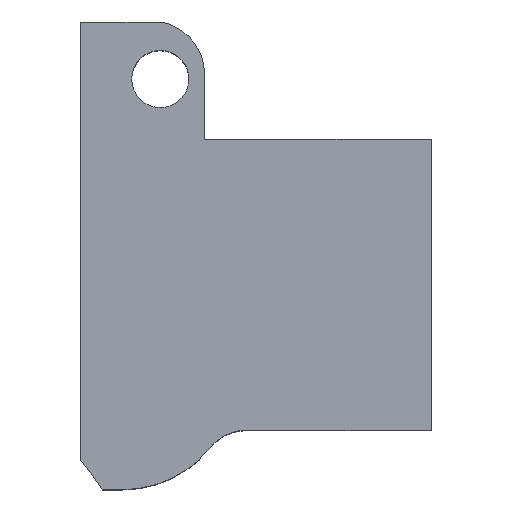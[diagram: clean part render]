
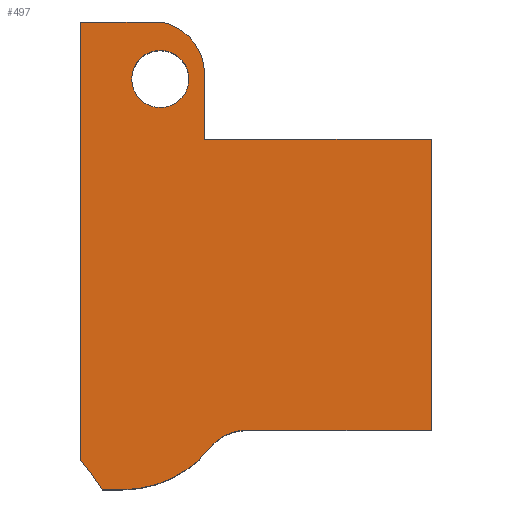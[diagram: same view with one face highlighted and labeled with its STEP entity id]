
A CAD part, top view. The second image highlights one B-rep face of the part: STEP entity #497.
In plain terms, the highlighted planar face has unit normal (0, 0, 1).
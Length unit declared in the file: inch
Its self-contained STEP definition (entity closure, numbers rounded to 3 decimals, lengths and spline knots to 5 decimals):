
#15 = FACE_OUTER_BOUND ( 'NONE', #800, .T. ) ;
#30 = CARTESIAN_POINT ( 'NONE',  ( 3.70038, -0.51472, 0.4665 ) ) ;
#53 = VERTEX_POINT ( 'NONE', #881 ) ;
#54 = CARTESIAN_POINT ( 'NONE',  ( 2.19337, -1.9664, 0.4665 ) ) ;
#58 = DIRECTION ( 'NONE',  ( 0., 0., -1. ) ) ;
#61 = DIRECTION ( 'NONE',  ( 0., -1., 0. ) ) ;
#66 = ORIENTED_EDGE ( 'NONE', *, *, #389, .T. ) ;
#77 = VECTOR ( 'NONE', #61, 39.37008 ) ;
#79 = AXIS2_PLACEMENT_3D ( 'NONE', #520, #877, #338 ) ;
#88 = ORIENTED_EDGE ( 'NONE', *, *, #397, .F. ) ;
#92 = ORIENTED_EDGE ( 'NONE', *, *, #427, .T. ) ;
#100 = LINE ( 'NONE', #954, #1010 ) ;
#102 = CARTESIAN_POINT ( 'NONE',  ( 2.6348, -0.2505, 0.4665 ) ) ;
#106 = CARTESIAN_POINT ( 'NONE',  ( 2.5093, -0.2505, 0.4665 ) ) ;
#114 = AXIS2_PLACEMENT_3D ( 'NONE', #1031, #531, #1122 ) ;
#127 = CARTESIAN_POINT ( 'NONE',  ( 2.3447, -2.0545, 0.4665 ) ) ;
#131 = AXIS2_PLACEMENT_3D ( 'NONE', #1025, #522, #1116 ) ;
#135 = CARTESIAN_POINT ( 'NONE',  ( 2.5093, -0.2505, 0.4665 ) ) ;
#141 = CARTESIAN_POINT ( 'NONE',  ( 2.22441, -2.00982, 0.4665 ) ) ;
#147 = AXIS2_PLACEMENT_3D ( 'NONE', #619, #58, #724 ) ;
#148 = AXIS2_PLACEMENT_3D ( 'NONE', #135, #789, #238 ) ;
#150 = DIRECTION ( 'NONE',  ( 0., 1., 0. ) ) ;
#157 = VECTOR ( 'NONE', #1098, 39.37008 ) ;
#163 = VERTEX_POINT ( 'NONE', #548 ) ;
#188 = LINE ( 'NONE', #712, #157 ) ;
#206 = DIRECTION ( 'NONE',  ( 1., 0., 0. ) ) ;
#207 = AXIS2_PLACEMENT_3D ( 'NONE', #106, #762, #206 ) ;
#227 = CARTESIAN_POINT ( 'NONE',  ( 2.3838, -0.2505, 0.4665 ) ) ;
#237 = FACE_BOUND ( 'NONE', #1029, .T. ) ;
#238 = DIRECTION ( 'NONE',  ( 1., 0., 0. ) ) ;
#244 = CARTESIAN_POINT ( 'NONE',  ( 2.25374, -2.0545, 0.4665 ) ) ;
#250 = CARTESIAN_POINT ( 'NONE',  ( -5.73341, -0.51472, 0.4665 ) ) ;
#293 = EDGE_CURVE ( 'NONE', #688, #894, #646, .T. ) ;
#309 = ORIENTED_EDGE ( 'NONE', *, *, #374, .T. ) ;
#314 = CIRCLE ( 'NONE', #114, 0.23133 ) ;
#338 = DIRECTION ( 'NONE',  ( 1., 0., 0. ) ) ;
#346 = LINE ( 'NONE', #872, #77 ) ;
#351 = VERTEX_POINT ( 'NONE', #398 ) ;
#368 = VECTOR ( 'NONE', #1107, 39.37008 ) ;
#373 = VERTEX_POINT ( 'NONE', #508 ) ;
#374 = EDGE_CURVE ( 'NONE', #894, #688, #396, .T. ) ;
#384 = EDGE_CURVE ( 'NONE', #791, #746, #188, .T. ) ;
#389 = EDGE_CURVE ( 'NONE', #791, #351, #1088, .T. ) ;
#390 = EDGE_CURVE ( 'NONE', #351, #605, #1068, .T. ) ;
#396 = CIRCLE ( 'NONE', #148, 0.1255 ) ;
#397 = EDGE_CURVE ( 'NONE', #995, #605, #634, .T. ) ;
#398 = CARTESIAN_POINT ( 'NONE',  ( 2.1593, -1.92524, 0.4665 ) ) ;
#399 = EDGE_CURVE ( 'NONE', #53, #995, #1062, .T. ) ;
#408 = EDGE_CURVE ( 'NONE', #53, #373, #831, .T. ) ;
#413 = CARTESIAN_POINT ( 'NONE',  ( 2.1593, -1.92524, 0.4665 ) ) ;
#418 = EDGE_CURVE ( 'NONE', #373, #860, #100, .T. ) ;
#421 = EDGE_CURVE ( 'NONE', #835, #860, #346, .T. ) ;
#426 = DIRECTION ( 'NONE',  ( 1., 0., 0. ) ) ;
#427 = EDGE_CURVE ( 'NONE', #835, #163, #782, .T. ) ;
#434 = EDGE_CURVE ( 'NONE', #163, #880, #989, .T. ) ;
#435 = EDGE_CURVE ( 'NONE', #746, #880, #314, .T. ) ;
#474 = ORIENTED_EDGE ( 'NONE', *, *, #421, .F. ) ;
#497 = ADVANCED_FACE ( 'NONE', ( #237, #15 ), #628, .T. ) ;
#508 = CARTESIAN_POINT ( 'NONE',  ( 2.8839, -1.79442, 0.4665 ) ) ;
#520 = CARTESIAN_POINT ( 'NONE',  ( -1.02672, -2.07217, 0.4665 ) ) ;
#522 = DIRECTION ( 'NONE',  ( 0., 0., -1. ) ) ;
#531 = DIRECTION ( 'NONE',  ( 0., 0., -1. ) ) ;
#532 = ORIENTED_EDGE ( 'NONE', *, *, #435, .F. ) ;
#543 = VECTOR ( 'NONE', #729, 39.37008 ) ;
#548 = CARTESIAN_POINT ( 'NONE',  ( 2.70341, -0.51472, 0.4665 ) ) ;
#550 = ORIENTED_EDGE ( 'NONE', *, *, #408, .T. ) ;
#605 = VERTEX_POINT ( 'NONE', #981 ) ;
#606 = DIRECTION ( 'NONE',  ( 0., -1., 0. ) ) ;
#613 = CARTESIAN_POINT ( 'NONE',  ( 2.17697, -1.94534, 0.4665 ) ) ;
#619 = CARTESIAN_POINT ( 'NONE',  ( 2.3447, -1.56238, 0.4665 ) ) ;
#626 = CARTESIAN_POINT ( 'NONE',  ( 2.70341, -2.62989, 0.4665 ) ) ;
#628 = PLANE ( 'NONE',  #79 ) ;
#634 = LINE ( 'NONE', #1020, #368 ) ;
#646 = CIRCLE ( 'NONE', #207, 0.1255 ) ;
#653 = ORIENTED_EDGE ( 'NONE', *, *, #399, .F. ) ;
#688 = VERTEX_POINT ( 'NONE', #102 ) ;
#689 = CARTESIAN_POINT ( 'NONE',  ( 2.1593, 0., 0.4665 ) ) ;
#712 = CARTESIAN_POINT ( 'NONE',  ( 2.5093, 0., 0.4665 ) ) ;
#719 = CARTESIAN_POINT ( 'NONE',  ( 2.20126, -1.97716, 0.4665 ) ) ;
#724 = DIRECTION ( 'NONE',  ( 1., 0., 0. ) ) ;
#729 = DIRECTION ( 'NONE',  ( -1., 0., 0. ) ) ;
#733 = ORIENTED_EDGE ( 'NONE', *, *, #293, .T. ) ;
#746 = VERTEX_POINT ( 'NONE', #841 ) ;
#762 = DIRECTION ( 'NONE',  ( 0., 0., -1. ) ) ;
#782 = LINE ( 'NONE', #250, #543 ) ;
#784 = CARTESIAN_POINT ( 'NONE',  ( 2.1593, -2.07217, 0.4665 ) ) ;
#789 = DIRECTION ( 'NONE',  ( 0., 0., -1. ) ) ;
#791 = VERTEX_POINT ( 'NONE', #689 ) ;
#793 = CARTESIAN_POINT ( 'NONE',  ( 2.2392, -2.03208, 0.4665 ) ) ;
#800 = EDGE_LOOP ( 'NONE', ( #1105, #66, #875, #88, #653, #550, #1123, #474, #92, #893, #532 ) ) ;
#809 = VECTOR ( 'NONE', #150, 39.37008 ) ;
#831 = CIRCLE ( 'NONE', #131, 0.19685 ) ;
#835 = VERTEX_POINT ( 'NONE', #30 ) ;
#841 = CARTESIAN_POINT ( 'NONE',  ( 2.5093, 0., 0.4665 ) ) ;
#852 = VECTOR ( 'NONE', #606, 39.37008 ) ;
#853 = CARTESIAN_POINT ( 'NONE',  ( 2.70341, -0.22831, 0.4665 ) ) ;
#860 = VERTEX_POINT ( 'NONE', #929 ) ;
#872 = CARTESIAN_POINT ( 'NONE',  ( 3.70038, 1.01705, 0.4665 ) ) ;
#875 = ORIENTED_EDGE ( 'NONE', *, *, #390, .T. ) ;
#877 = DIRECTION ( 'NONE',  ( 0., 0., 1. ) ) ;
#880 = VERTEX_POINT ( 'NONE', #853 ) ;
#881 = CARTESIAN_POINT ( 'NONE',  ( 2.72984, -1.86873, 0.4665 ) ) ;
#893 = ORIENTED_EDGE ( 'NONE', *, *, #434, .T. ) ;
#894 = VERTEX_POINT ( 'NONE', #227 ) ;
#929 = CARTESIAN_POINT ( 'NONE',  ( 3.70038, -1.79442, 0.4665 ) ) ;
#943 = CARTESIAN_POINT ( 'NONE',  ( 2.16848, -1.93503, 0.4665 ) ) ;
#954 = CARTESIAN_POINT ( 'NONE',  ( -1.85818, -1.79442, 0.4665 ) ) ;
#981 = CARTESIAN_POINT ( 'NONE',  ( 2.25374, -2.0545, 0.4665 ) ) ;
#989 = LINE ( 'NONE', #626, #809 ) ;
#995 = VERTEX_POINT ( 'NONE', #127 ) ;
#1010 = VECTOR ( 'NONE', #426, 39.37008 ) ;
#1020 = CARTESIAN_POINT ( 'NONE',  ( 0., -2.0545, 0.4665 ) ) ;
#1025 = CARTESIAN_POINT ( 'NONE',  ( 2.8839, -1.99127, 0.4665 ) ) ;
#1029 = EDGE_LOOP ( 'NONE', ( #733, #309 ) ) ;
#1031 = CARTESIAN_POINT ( 'NONE',  ( 2.47208, -0.22831, 0.4665 ) ) ;
#1062 = CIRCLE ( 'NONE', #147, 0.49213 ) ;
#1068 = B_SPLINE_CURVE_WITH_KNOTS ( 'NONE', 3,
 ( #413, #943, #613, #54, #719, #141, #793, #244 ),
 .UNSPECIFIED., .F., .F.,
 ( 4, 2, 2, 4 ),
 ( 0., 0.00102, 0.00203, 0.00407 ),
 .UNSPECIFIED. ) ;
#1088 = LINE ( 'NONE', #784, #852 ) ;
#1098 = DIRECTION ( 'NONE',  ( 1., 0., 0. ) ) ;
#1105 = ORIENTED_EDGE ( 'NONE', *, *, #384, .F. ) ;
#1107 = DIRECTION ( 'NONE',  ( -1., 0., 0. ) ) ;
#1116 = DIRECTION ( 'NONE',  ( 1., 0., 0. ) ) ;
#1122 = DIRECTION ( 'NONE',  ( 1., 0., 0. ) ) ;
#1123 = ORIENTED_EDGE ( 'NONE', *, *, #418, .T. ) ;
